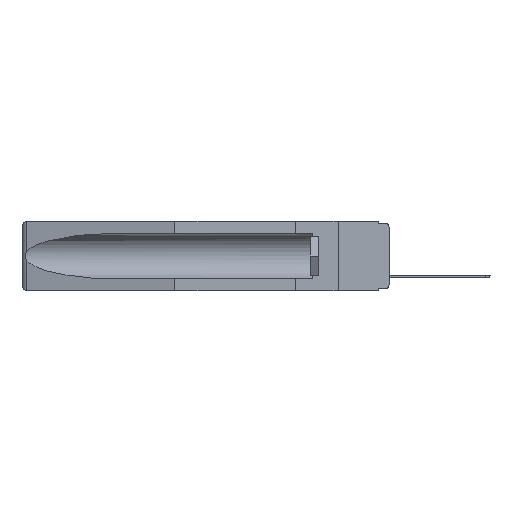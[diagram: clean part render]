
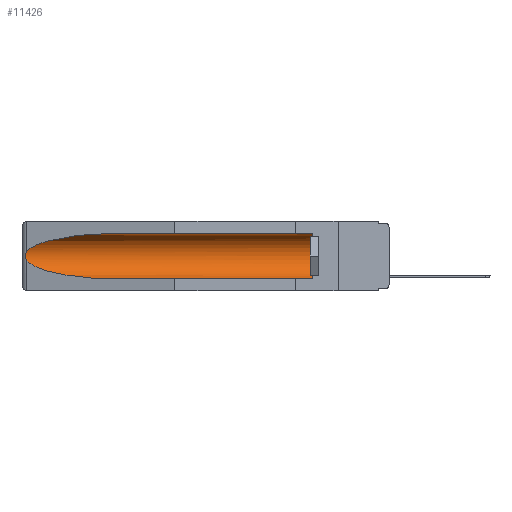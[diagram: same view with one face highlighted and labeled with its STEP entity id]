
A CAD part, left-side view. The second image highlights one B-rep face of the part: STEP entity #11426.
In plain terms, the highlighted cylindrical face has radius 2.857 mm (diameter 5.715 mm), a partial arc.
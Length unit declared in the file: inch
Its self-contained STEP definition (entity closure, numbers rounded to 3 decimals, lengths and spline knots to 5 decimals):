
#180 = ORIENTED_EDGE ( 'NONE', *, *, #1818, .T. ) ;
#921 = CYLINDRICAL_SURFACE ( 'NONE', #2006, 0.1125 ) ;
#1818 = EDGE_CURVE ( 'NONE', #14736, #23709, #21469, .T. ) ;
#2006 = AXIS2_PLACEMENT_3D ( 'NONE', #18808, #24646, #18303 ) ;
#2095 = DIRECTION ( 'NONE',  ( 0., 1., 0. ) ) ;
#2358 = ORIENTED_EDGE ( 'NONE', *, *, #21177, .F. ) ;
#2414 = CARTESIAN_POINT ( 'NONE',  ( 0.2673, 1.53269, -0.17917 ) ) ;
#2545 = CARTESIAN_POINT ( 'NONE',  ( 0.26654, 1.53092, -0.15636 ) ) ;
#2875 = VERTEX_POINT ( 'NONE', #17291 ) ;
#4418 = CARTESIAN_POINT ( 'NONE',  ( 0.155, 1.07973, -0.059 ) ) ;
#4511 = CARTESIAN_POINT ( 'NONE',  ( 0.155, 1.07973, -0.284 ) ) ;
#5382 = EDGE_CURVE ( 'NONE', #9781, #21017, #17072, .T. ) ;
#5871 = ORIENTED_EDGE ( 'NONE', *, *, #11407, .T. ) ;
#6073 = ORIENTED_EDGE ( 'NONE', *, *, #5382, .T. ) ;
#6367 = CARTESIAN_POINT ( 'NONE',  ( 0.26597, 1.52961, -0.15275 ) ) ;
#8003 = CARTESIAN_POINT ( 'NONE',  ( 0.26537, 1.52718, -0.19328 ) ) ;
#8404 = CARTESIAN_POINT ( 'NONE',  ( 0.2673, 1.5327, -0.16383 ) ) ;
#8634 = CARTESIAN_POINT ( 'NONE',  ( 0.26537, 1.52718, -0.14972 ) ) ;
#9002 = DIRECTION ( 'NONE',  ( 0., 0., 1. ) ) ;
#9157 = CIRCLE ( 'NONE', #21792, 0.1125 ) ;
#9417 = CARTESIAN_POINT ( 'NONE',  ( 0.26537, 1.52718, -0.19328 ) ) ;
#9781 = VERTEX_POINT ( 'NONE', #21002 ) ;
#10183 = CARTESIAN_POINT ( 'NONE',  ( 0.26537, 1.52718, -0.19328 ) ) ;
#11407 = EDGE_CURVE ( 'NONE', #21017, #14736, #13157, .T. ) ;
#11426 = ADVANCED_FACE ( 'NONE', ( #14844 ), #921, .F. ) ;
#11604 = CARTESIAN_POINT ( 'NONE',  ( 0.155, 1.07973, -0.284 ) ) ;
#11795 = LINE ( 'NONE', #23425, #19575 ) ;
#13084 = DIRECTION ( 'NONE',  ( 0., 1., 0. ) ) ;
#13157 =( BOUNDED_CURVE ( )  B_SPLINE_CURVE ( 3, ( #14711, #16644, #16903, #22724 ),
 .UNSPECIFIED., .F., .F. ) 
 B_SPLINE_CURVE_WITH_KNOTS ( ( 4, 4 ),
 ( 4.71239, 6.08839 ),
 .UNSPECIFIED. ) 
 CURVE ( )  GEOMETRIC_REPRESENTATION_ITEM ( )  RATIONAL_B_SPLINE_CURVE ( ( 1., 0.848, 0.848, 1. ) ) 
 REPRESENTATION_ITEM ( '' )  );
#13310 = VECTOR ( 'NONE', #13084, 39.37008 ) ;
#13336 = ORIENTED_EDGE ( 'NONE', *, *, #24896, .T. ) ;
#14308 = CARTESIAN_POINT ( 'NONE',  ( 0.26597, 1.5296, -0.19026 ) ) ;
#14711 = CARTESIAN_POINT ( 'NONE',  ( 0.155, 1.07973, -0.059 ) ) ;
#14736 = VERTEX_POINT ( 'NONE', #8634 ) ;
#14844 = FACE_OUTER_BOUND ( 'NONE', #19871, .T. ) ;
#16113 = CARTESIAN_POINT ( 'NONE',  ( 0.26537, 1.52718, -0.14972 ) ) ;
#16232 = CARTESIAN_POINT ( 'NONE',  ( 0.2675, 1.53308, -0.17534 ) ) ;
#16644 = CARTESIAN_POINT ( 'NONE',  ( 0.21114, 1.30732, -0.059 ) ) ;
#16903 = CARTESIAN_POINT ( 'NONE',  ( 0.25451, 1.48313, -0.09465 ) ) ;
#17072 = LINE ( 'NONE', #24811, #13310 ) ;
#17291 = CARTESIAN_POINT ( 'NONE',  ( 0.155, 0.126, -0.284 ) ) ;
#17346 = CARTESIAN_POINT ( 'NONE',  ( 0.155, 0.126, -0.1715 ) ) ;
#17925 = EDGE_CURVE ( 'NONE', #2875, #9781, #9157, .T. ) ;
#18303 = DIRECTION ( 'NONE',  ( 0., 0., 1. ) ) ;
#18808 = CARTESIAN_POINT ( 'NONE',  ( 0.155, -0.30754, -0.1715 ) ) ;
#19575 = VECTOR ( 'NONE', #2095, 39.37008 ) ;
#19871 = EDGE_LOOP ( 'NONE', ( #5871, #180, #13336, #2358, #23023, #6073 ) ) ;
#19910 = CARTESIAN_POINT ( 'NONE',  ( 0.2675, 1.53308, -0.16763 ) ) ;
#20761 = DIRECTION ( 'NONE',  ( 0., -1., 0. ) ) ;
#20934 = CARTESIAN_POINT ( 'NONE',  ( 0.25451, 1.48313, -0.24835 ) ) ;
#21002 = CARTESIAN_POINT ( 'NONE',  ( 0.155, 0.126, -0.059 ) ) ;
#21017 = VERTEX_POINT ( 'NONE', #4418 ) ;
#21177 = EDGE_CURVE ( 'NONE', #2875, #21351, #11795, .T. ) ;
#21351 = VERTEX_POINT ( 'NONE', #4511 ) ;
#21469 = B_SPLINE_CURVE_WITH_KNOTS ( 'NONE', 3,
 ( #16113, #6367, #2545, #8404, #19910, #16232, #2414, #23980, #14308, #10183 ),
 .UNSPECIFIED., .F., .F.,
 ( 4, 2, 2, 2, 4 ),
 ( 0., 0.00029, 0.00058, 0.00087, 0.00117 ),
 .UNSPECIFIED. ) ;
#21792 = AXIS2_PLACEMENT_3D ( 'NONE', #17346, #20761, #9002 ) ;
#22724 = CARTESIAN_POINT ( 'NONE',  ( 0.26537, 1.52718, -0.14972 ) ) ;
#22804 =( BOUNDED_CURVE ( )  B_SPLINE_CURVE ( 3, ( #9417, #20934, #25006, #11604 ),
 .UNSPECIFIED., .F., .F. ) 
 B_SPLINE_CURVE_WITH_KNOTS ( ( 4, 4 ),
 ( 0.1948, 1.5708 ),
 .UNSPECIFIED. ) 
 CURVE ( )  GEOMETRIC_REPRESENTATION_ITEM ( )  RATIONAL_B_SPLINE_CURVE ( ( 1., 0.848, 0.848, 1. ) ) 
 REPRESENTATION_ITEM ( '' )  );
#23023 = ORIENTED_EDGE ( 'NONE', *, *, #17925, .T. ) ;
#23425 = CARTESIAN_POINT ( 'NONE',  ( 0.155, -0.30754, -0.284 ) ) ;
#23709 = VERTEX_POINT ( 'NONE', #8003 ) ;
#23980 = CARTESIAN_POINT ( 'NONE',  ( 0.26655, 1.53094, -0.18657 ) ) ;
#24646 = DIRECTION ( 'NONE',  ( 0., 1., 0. ) ) ;
#24811 = CARTESIAN_POINT ( 'NONE',  ( 0.155, -0.30754, -0.059 ) ) ;
#24896 = EDGE_CURVE ( 'NONE', #23709, #21351, #22804, .T. ) ;
#25006 = CARTESIAN_POINT ( 'NONE',  ( 0.21114, 1.30732, -0.284 ) ) ;
